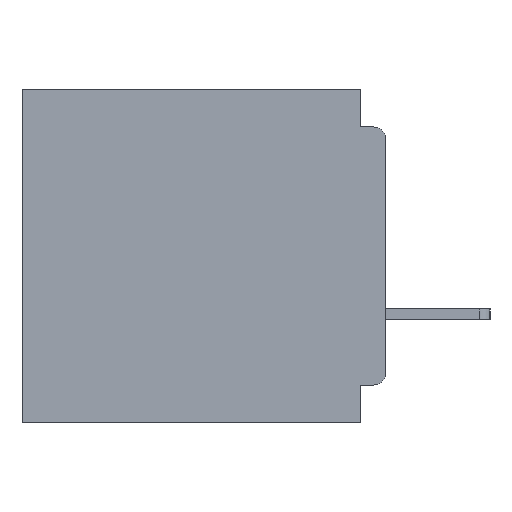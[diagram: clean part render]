
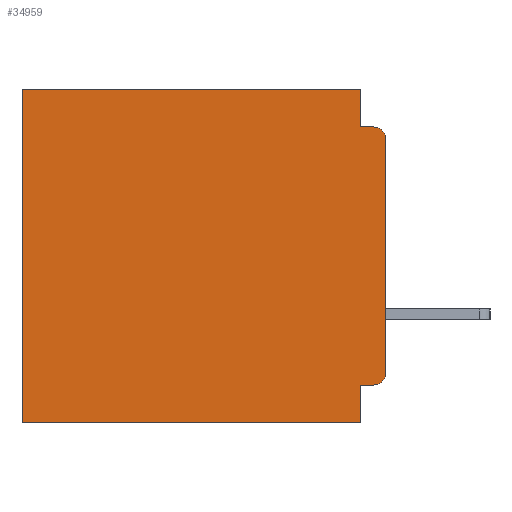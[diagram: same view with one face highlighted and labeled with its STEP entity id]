
A CAD part, left-side view. The second image highlights one B-rep face of the part: STEP entity #34959.
In plain terms, the highlighted planar face has unit normal (-1, 0, 0).
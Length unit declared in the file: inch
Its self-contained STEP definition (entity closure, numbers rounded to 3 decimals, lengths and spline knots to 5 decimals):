
#648 = VERTEX_POINT ( 'NONE', #11582 ) ;
#749 = DIRECTION ( 'NONE',  ( 0., -1., 0. ) ) ;
#755 = CARTESIAN_POINT ( 'NONE',  ( 0.3, 0., -0.06 ) ) ;
#1748 = DIRECTION ( 'NONE',  ( 0., 0., -1. ) ) ;
#2658 = ORIENTED_EDGE ( 'NONE', *, *, #20105, .F. ) ;
#4629 = CARTESIAN_POINT ( 'NONE',  ( 0.3, 0.031, -0.4 ) ) ;
#4788 = ORIENTED_EDGE ( 'NONE', *, *, #31040, .T. ) ;
#5231 = VECTOR ( 'NONE', #16400, 39.37008 ) ;
#6586 = LINE ( 'NONE', #20087, #41228 ) ;
#9130 = ORIENTED_EDGE ( 'NONE', *, *, #33007, .F. ) ;
#11582 = CARTESIAN_POINT ( 'NONE',  ( 0.3, 0.437, -0.4 ) ) ;
#11901 = CARTESIAN_POINT ( 'NONE',  ( 0.3, 0.031, -0.045 ) ) ;
#11995 = CIRCLE ( 'NONE', #15401, 0.015 ) ;
#12164 = DIRECTION ( 'NONE',  ( 1., 0., 0. ) ) ;
#12459 = EDGE_CURVE ( 'NONE', #36373, #56538, #15676, .T. ) ;
#14223 = EDGE_CURVE ( 'NONE', #37531, #52259, #17430, .T. ) ;
#14631 = CARTESIAN_POINT ( 'NONE',  ( 0.3, 0., -0.045 ) ) ;
#14741 = LINE ( 'NONE', #14631, #49260 ) ;
#14778 = DIRECTION ( 'NONE',  ( 0., 1., 0. ) ) ;
#15401 = AXIS2_PLACEMENT_3D ( 'NONE', #23358, #54786, #27856 ) ;
#15605 = CARTESIAN_POINT ( 'NONE',  ( 0.3, 0.437, 0. ) ) ;
#15676 = LINE ( 'NONE', #17240, #51577 ) ;
#16035 = CARTESIAN_POINT ( 'NONE',  ( 0.3, 0.015, -0.34 ) ) ;
#16400 = DIRECTION ( 'NONE',  ( 0., 1., 0. ) ) ;
#16566 = CARTESIAN_POINT ( 'NONE',  ( 0.3, 0., -0.4 ) ) ;
#17240 = CARTESIAN_POINT ( 'NONE',  ( 0.3, 0.031, -0.4 ) ) ;
#17430 = LINE ( 'NONE', #20916, #5231 ) ;
#20087 = CARTESIAN_POINT ( 'NONE',  ( 0.3, 0., -0.4 ) ) ;
#20105 = EDGE_CURVE ( 'NONE', #29996, #36373, #46721, .T. ) ;
#20400 = VECTOR ( 'NONE', #23827, 39.37008 ) ;
#20540 = DIRECTION ( 'NONE',  ( 0., 0., -1. ) ) ;
#20916 = CARTESIAN_POINT ( 'NONE',  ( 0.3, 0., 0. ) ) ;
#23358 = CARTESIAN_POINT ( 'NONE',  ( 0.3, 0.015, -0.06 ) ) ;
#23827 = DIRECTION ( 'NONE',  ( 0., 0., -1. ) ) ;
#24653 = DIRECTION ( 'NONE',  ( 0., 1., 0. ) ) ;
#26199 = VERTEX_POINT ( 'NONE', #41690 ) ;
#26992 = AXIS2_PLACEMENT_3D ( 'NONE', #16035, #47474, #20540 ) ;
#27371 = EDGE_CURVE ( 'NONE', #30535, #49425, #14741, .T. ) ;
#27856 = DIRECTION ( 'NONE',  ( 0., 0., -1. ) ) ;
#29001 = CARTESIAN_POINT ( 'NONE',  ( 0.3, 0.437, -0.4 ) ) ;
#29306 = CARTESIAN_POINT ( 'NONE',  ( 0.3, 0.015, -0.355 ) ) ;
#29389 = AXIS2_PLACEMENT_3D ( 'NONE', #16566, #12164, #43684 ) ;
#29996 = VERTEX_POINT ( 'NONE', #29306 ) ;
#30529 = VECTOR ( 'NONE', #50808, 39.37008 ) ;
#30535 = VERTEX_POINT ( 'NONE', #11901 ) ;
#30958 = CARTESIAN_POINT ( 'NONE',  ( 0.3, 0.031, -0.355 ) ) ;
#31040 = EDGE_CURVE ( 'NONE', #52259, #648, #43829, .T. ) ;
#32393 = ORIENTED_EDGE ( 'NONE', *, *, #27371, .F. ) ;
#33007 = EDGE_CURVE ( 'NONE', #56538, #648, #6586, .T. ) ;
#33126 = ORIENTED_EDGE ( 'NONE', *, *, #12459, .F. ) ;
#34675 = VECTOR ( 'NONE', #1748, 39.37008 ) ;
#34758 = VECTOR ( 'NONE', #14778, 39.37008 ) ;
#34959 = ADVANCED_FACE ( 'NONE', ( #40292 ), #39161, .F. ) ;
#36373 = VERTEX_POINT ( 'NONE', #30958 ) ;
#37217 = EDGE_CURVE ( 'NONE', #37531, #30535, #42941, .T. ) ;
#37328 = ORIENTED_EDGE ( 'NONE', *, *, #45485, .F. ) ;
#37396 = CARTESIAN_POINT ( 'NONE',  ( 0.3, 0., -0.4 ) ) ;
#37531 = VERTEX_POINT ( 'NONE', #57760 ) ;
#38772 = ORIENTED_EDGE ( 'NONE', *, *, #47126, .T. ) ;
#38826 = ORIENTED_EDGE ( 'NONE', *, *, #40708, .T. ) ;
#39161 = PLANE ( 'NONE',  #29389 ) ;
#40292 = FACE_OUTER_BOUND ( 'NONE', #49278, .T. ) ;
#40708 = EDGE_CURVE ( 'NONE', #29996, #26199, #51760, .T. ) ;
#40812 = CARTESIAN_POINT ( 'NONE',  ( 0.3, 0.015, -0.045 ) ) ;
#41228 = VECTOR ( 'NONE', #24653, 39.37008 ) ;
#41690 = CARTESIAN_POINT ( 'NONE',  ( 0.3, 0., -0.34 ) ) ;
#41718 = CARTESIAN_POINT ( 'NONE',  ( 0.3, 0., -0.355 ) ) ;
#42522 = LINE ( 'NONE', #37396, #30529 ) ;
#42941 = LINE ( 'NONE', #50758, #20400 ) ;
#43684 = DIRECTION ( 'NONE',  ( 0., 0., -1. ) ) ;
#43829 = LINE ( 'NONE', #29001, #34675 ) ;
#44932 = VERTEX_POINT ( 'NONE', #755 ) ;
#45485 = EDGE_CURVE ( 'NONE', #44932, #26199, #42522, .T. ) ;
#46721 = LINE ( 'NONE', #41718, #34758 ) ;
#47126 = EDGE_CURVE ( 'NONE', #44932, #49425, #11995, .T. ) ;
#47474 = DIRECTION ( 'NONE',  ( -1., 0., 0. ) ) ;
#49260 = VECTOR ( 'NONE', #749, 39.37008 ) ;
#49278 = EDGE_LOOP ( 'NONE', ( #37328, #38772, #32393, #50062, #51493, #4788, #9130, #33126, #2658, #38826 ) ) ;
#49425 = VERTEX_POINT ( 'NONE', #40812 ) ;
#50062 = ORIENTED_EDGE ( 'NONE', *, *, #37217, .F. ) ;
#50758 = CARTESIAN_POINT ( 'NONE',  ( 0.3, 0.031, 0. ) ) ;
#50808 = DIRECTION ( 'NONE',  ( 0., 0., -1. ) ) ;
#51493 = ORIENTED_EDGE ( 'NONE', *, *, #14223, .T. ) ;
#51577 = VECTOR ( 'NONE', #53021, 39.37008 ) ;
#51760 = CIRCLE ( 'NONE', #26992, 0.015 ) ;
#52259 = VERTEX_POINT ( 'NONE', #15605 ) ;
#53021 = DIRECTION ( 'NONE',  ( 0., 0., -1. ) ) ;
#54786 = DIRECTION ( 'NONE',  ( -1., 0., 0. ) ) ;
#56538 = VERTEX_POINT ( 'NONE', #4629 ) ;
#57760 = CARTESIAN_POINT ( 'NONE',  ( 0.3, 0.031, 0. ) ) ;
